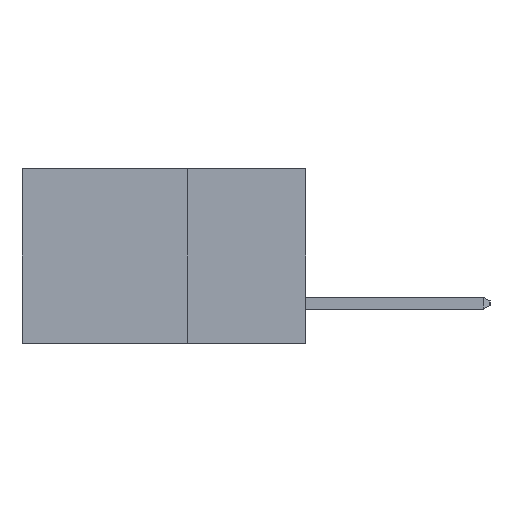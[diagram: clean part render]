
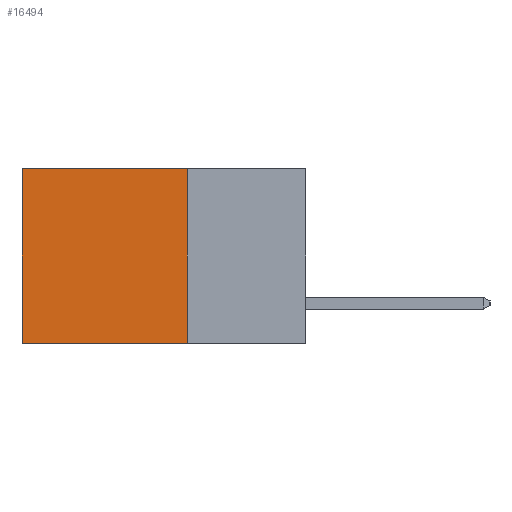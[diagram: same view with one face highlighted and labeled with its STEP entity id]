
A CAD part, left-side view. The second image highlights one B-rep face of the part: STEP entity #16494.
In plain terms, the highlighted planar face has unit normal (-1, 0, 0).
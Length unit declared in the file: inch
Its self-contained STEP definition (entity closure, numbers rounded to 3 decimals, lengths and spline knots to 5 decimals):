
#342 = VECTOR ( 'NONE', #23884, 39.37008 ) ;
#573 = CARTESIAN_POINT ( 'NONE',  ( 0.298, 0.6, 0. ) ) ;
#1035 = VERTEX_POINT ( 'NONE', #7880 ) ;
#1524 = CARTESIAN_POINT ( 'NONE',  ( 0.298, 0.25, 0. ) ) ;
#1563 = LINE ( 'NONE', #4169, #21061 ) ;
#1792 = DIRECTION ( 'NONE',  ( 0., 0., -1. ) ) ;
#2734 = VERTEX_POINT ( 'NONE', #573 ) ;
#2758 = EDGE_CURVE ( 'NONE', #2734, #1035, #10027, .T. ) ;
#3315 = CARTESIAN_POINT ( 'NONE',  ( 0.298, 0.25, 0. ) ) ;
#4169 = CARTESIAN_POINT ( 'NONE',  ( 0.298, 0.25, 0. ) ) ;
#5402 = DIRECTION ( 'NONE',  ( 1., 0., 0. ) ) ;
#5529 = LINE ( 'NONE', #3315, #342 ) ;
#7421 = EDGE_CURVE ( 'NONE', #16613, #1035, #23493, .T. ) ;
#7556 = CARTESIAN_POINT ( 'NONE',  ( 0.298, 0.6, 0. ) ) ;
#7880 = CARTESIAN_POINT ( 'NONE',  ( 0.298, 0.6, -0.37 ) ) ;
#8860 = EDGE_CURVE ( 'NONE', #15391, #2734, #5529, .T. ) ;
#9507 = CARTESIAN_POINT ( 'NONE',  ( 0.298, 0.25, -0.37 ) ) ;
#9732 = DIRECTION ( 'NONE',  ( 0., 1., 0. ) ) ;
#10027 = LINE ( 'NONE', #7556, #19408 ) ;
#11706 = ORIENTED_EDGE ( 'NONE', *, *, #8860, .T. ) ;
#13182 = CARTESIAN_POINT ( 'NONE',  ( 0.298, 0.25, -0.37 ) ) ;
#13665 = ORIENTED_EDGE ( 'NONE', *, *, #7421, .F. ) ;
#15391 = VERTEX_POINT ( 'NONE', #20976 ) ;
#16494 = ADVANCED_FACE ( 'NONE', ( #20185 ), #16719, .F. ) ;
#16613 = VERTEX_POINT ( 'NONE', #13182 ) ;
#16719 = PLANE ( 'NONE',  #17236 ) ;
#17236 = AXIS2_PLACEMENT_3D ( 'NONE', #1524, #5402, #18594 ) ;
#18484 = ORIENTED_EDGE ( 'NONE', *, *, #2758, .T. ) ;
#18586 = VECTOR ( 'NONE', #9732, 39.37008 ) ;
#18594 = DIRECTION ( 'NONE',  ( 0., 0., -1. ) ) ;
#19408 = VECTOR ( 'NONE', #1792, 39.37008 ) ;
#19767 = ORIENTED_EDGE ( 'NONE', *, *, #23312, .F. ) ;
#20185 = FACE_OUTER_BOUND ( 'NONE', #23056, .T. ) ;
#20976 = CARTESIAN_POINT ( 'NONE',  ( 0.298, 0.25, 0. ) ) ;
#21061 = VECTOR ( 'NONE', #22901, 39.37008 ) ;
#22901 = DIRECTION ( 'NONE',  ( 0., 0., -1. ) ) ;
#23056 = EDGE_LOOP ( 'NONE', ( #18484, #13665, #19767, #11706 ) ) ;
#23312 = EDGE_CURVE ( 'NONE', #15391, #16613, #1563, .T. ) ;
#23493 = LINE ( 'NONE', #9507, #18586 ) ;
#23884 = DIRECTION ( 'NONE',  ( 0., 1., 0. ) ) ;
